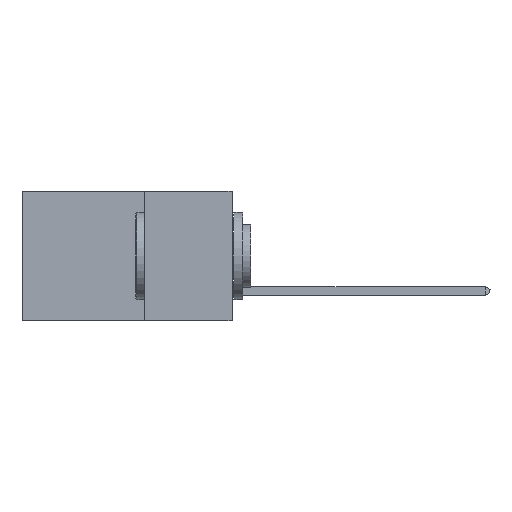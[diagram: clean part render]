
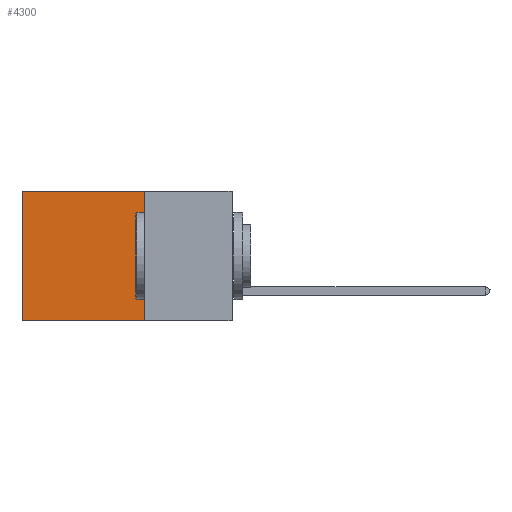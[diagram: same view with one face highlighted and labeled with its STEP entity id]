
A CAD part, left-side view. The second image highlights one B-rep face of the part: STEP entity #4300.
In plain terms, the highlighted planar face has unit normal (-1, 0, 0).
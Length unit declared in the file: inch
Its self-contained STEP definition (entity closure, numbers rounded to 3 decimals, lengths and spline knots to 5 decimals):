
#61 = LINE ( 'NONE', #32788, #22398 ) ;
#326 = VECTOR ( 'NONE', #26390, 39.37008 ) ;
#1720 = ORIENTED_EDGE ( 'NONE', *, *, #24578, .F. ) ;
#2339 = EDGE_CURVE ( 'NONE', #18174, #29328, #17586, .T. ) ;
#4300 = ADVANCED_FACE ( 'NONE', ( #31724 ), #5132, .F. ) ;
#5132 = PLANE ( 'NONE',  #8736 ) ;
#5271 = CARTESIAN_POINT ( 'NONE',  ( 0.2875, 0.25, 0. ) ) ;
#7959 = CARTESIAN_POINT ( 'NONE',  ( 0.2875, 0.25, -0.37 ) ) ;
#8391 = DIRECTION ( 'NONE',  ( 0., 0., -1. ) ) ;
#8736 = AXIS2_PLACEMENT_3D ( 'NONE', #21498, #37203, #8391 ) ;
#8971 = LINE ( 'NONE', #23670, #326 ) ;
#16556 = CARTESIAN_POINT ( 'NONE',  ( 0.2875, 0.6, -0.37 ) ) ;
#17586 = LINE ( 'NONE', #5271, #25729 ) ;
#18174 = VERTEX_POINT ( 'NONE', #33435 ) ;
#19406 = ORIENTED_EDGE ( 'NONE', *, *, #2339, .T. ) ;
#19656 = LINE ( 'NONE', #31828, #39884 ) ;
#21498 = CARTESIAN_POINT ( 'NONE',  ( 0.2875, 0.25, 0. ) ) ;
#22398 = VECTOR ( 'NONE', #29816, 39.37008 ) ;
#23084 = EDGE_LOOP ( 'NONE', ( #30521, #1720, #40779, #19406 ) ) ;
#23670 = CARTESIAN_POINT ( 'NONE',  ( 0.2875, 0.6, 0. ) ) ;
#24578 = EDGE_CURVE ( 'NONE', #33716, #38045, #61, .T. ) ;
#25729 = VECTOR ( 'NONE', #37645, 39.37008 ) ;
#26390 = DIRECTION ( 'NONE',  ( 0., 0., -1. ) ) ;
#29328 = VERTEX_POINT ( 'NONE', #35752 ) ;
#29816 = DIRECTION ( 'NONE',  ( 0., 1., 0. ) ) ;
#30521 = ORIENTED_EDGE ( 'NONE', *, *, #37942, .T. ) ;
#31724 = FACE_OUTER_BOUND ( 'NONE', #23084, .T. ) ;
#31828 = CARTESIAN_POINT ( 'NONE',  ( 0.2875, 0.25, 0. ) ) ;
#32788 = CARTESIAN_POINT ( 'NONE',  ( 0.2875, 0.25, -0.37 ) ) ;
#33435 = CARTESIAN_POINT ( 'NONE',  ( 0.2875, 0.25, 0. ) ) ;
#33716 = VERTEX_POINT ( 'NONE', #7959 ) ;
#35752 = CARTESIAN_POINT ( 'NONE',  ( 0.2875, 0.6, 0. ) ) ;
#37203 = DIRECTION ( 'NONE',  ( 1., 0., 0. ) ) ;
#37645 = DIRECTION ( 'NONE',  ( 0., 1., 0. ) ) ;
#37942 = EDGE_CURVE ( 'NONE', #29328, #38045, #8971, .T. ) ;
#38045 = VERTEX_POINT ( 'NONE', #16556 ) ;
#38442 = DIRECTION ( 'NONE',  ( 0., 0., -1. ) ) ;
#38478 = EDGE_CURVE ( 'NONE', #18174, #33716, #19656, .T. ) ;
#39884 = VECTOR ( 'NONE', #38442, 39.37008 ) ;
#40779 = ORIENTED_EDGE ( 'NONE', *, *, #38478, .F. ) ;
